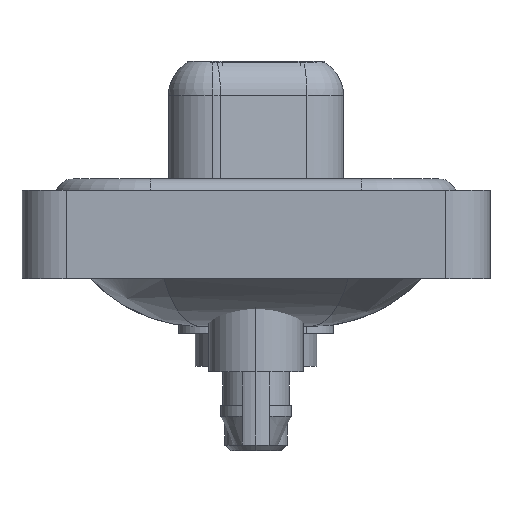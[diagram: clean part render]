
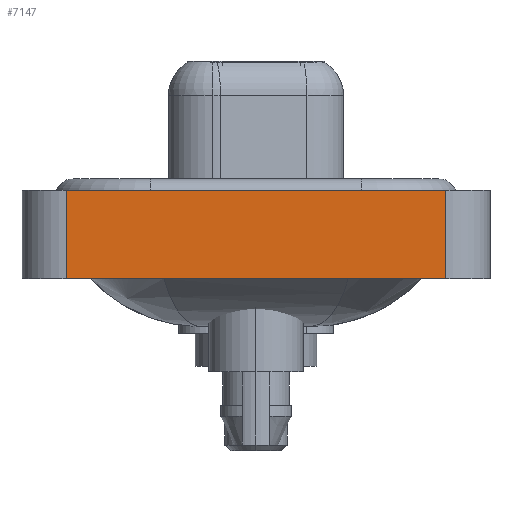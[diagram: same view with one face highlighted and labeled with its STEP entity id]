
A CAD part, left-side view. The second image highlights one B-rep face of the part: STEP entity #7147.
In plain terms, the highlighted planar face has unit normal (-1, 0, 0).
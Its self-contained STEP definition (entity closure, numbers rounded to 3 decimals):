
#234 = AXIS2_PLACEMENT_3D ( 'NONE', #5907, #10208, #10004 ) ;
#926 = LINE ( 'NONE', #2269, #4308 ) ;
#1220 = CARTESIAN_POINT ( 'NONE',  ( -7.3, 8.55, -3.6 ) ) ;
#2269 = CARTESIAN_POINT ( 'NONE',  ( -7.3, -8.55, 0.4 ) ) ;
#2755 = DIRECTION ( 'NONE',  ( 0., 0., 1. ) ) ;
#3711 = DIRECTION ( 'NONE',  ( 0., -1., 0. ) ) ;
#4308 = VECTOR ( 'NONE', #3711, 1000. ) ;
#4825 = VECTOR ( 'NONE', #8466, 1000. ) ;
#5907 = CARTESIAN_POINT ( 'NONE',  ( -7.3, -8.55, -3.6 ) ) ;
#6142 = ORIENTED_EDGE ( 'NONE', *, *, #7067, .T. ) ;
#7067 = EDGE_CURVE ( 'NONE', #12235, #18819, #17262, .T. ) ;
#7147 = ADVANCED_FACE ( 'NONE', ( #13181 ), #8599, .T. ) ;
#7220 = LINE ( 'NONE', #18877, #4825 ) ;
#7632 = EDGE_CURVE ( 'NONE', #18127, #18153, #7220, .T. ) ;
#7807 = ORIENTED_EDGE ( 'NONE', *, *, #15009, .F. ) ;
#8446 = EDGE_LOOP ( 'NONE', ( #6142, #7807, #17937, #16585 ) ) ;
#8466 = DIRECTION ( 'NONE',  ( 0., 0., 1. ) ) ;
#8586 = LINE ( 'NONE', #17546, #16142 ) ;
#8599 = PLANE ( 'NONE',  #234 ) ;
#10004 = DIRECTION ( 'NONE',  ( 0., 0., 1. ) ) ;
#10208 = DIRECTION ( 'NONE',  ( -1., 0., 0. ) ) ;
#10612 = VECTOR ( 'NONE', #2755, 1000. ) ;
#12235 = VERTEX_POINT ( 'NONE', #14776 ) ;
#13181 = FACE_OUTER_BOUND ( 'NONE', #8446, .T. ) ;
#14291 = CARTESIAN_POINT ( 'NONE',  ( -7.3, 8.55, 0.4 ) ) ;
#14776 = CARTESIAN_POINT ( 'NONE',  ( -7.3, -8.55, -3.6 ) ) ;
#15009 = EDGE_CURVE ( 'NONE', #18153, #18819, #926, .T. ) ;
#15733 = CARTESIAN_POINT ( 'NONE',  ( -7.3, -8.55, -3.6 ) ) ;
#16142 = VECTOR ( 'NONE', #18891, 1000. ) ;
#16585 = ORIENTED_EDGE ( 'NONE', *, *, #18128, .T. ) ;
#17262 = LINE ( 'NONE', #15733, #10612 ) ;
#17388 = CARTESIAN_POINT ( 'NONE',  ( -7.3, -8.55, 0.4 ) ) ;
#17546 = CARTESIAN_POINT ( 'NONE',  ( -7.3, -8.55, -3.6 ) ) ;
#17937 = ORIENTED_EDGE ( 'NONE', *, *, #7632, .F. ) ;
#18127 = VERTEX_POINT ( 'NONE', #1220 ) ;
#18128 = EDGE_CURVE ( 'NONE', #18127, #12235, #8586, .T. ) ;
#18153 = VERTEX_POINT ( 'NONE', #14291 ) ;
#18819 = VERTEX_POINT ( 'NONE', #17388 ) ;
#18877 = CARTESIAN_POINT ( 'NONE',  ( -7.3, 8.55, -3.6 ) ) ;
#18891 = DIRECTION ( 'NONE',  ( 0., -1., 0. ) ) ;
